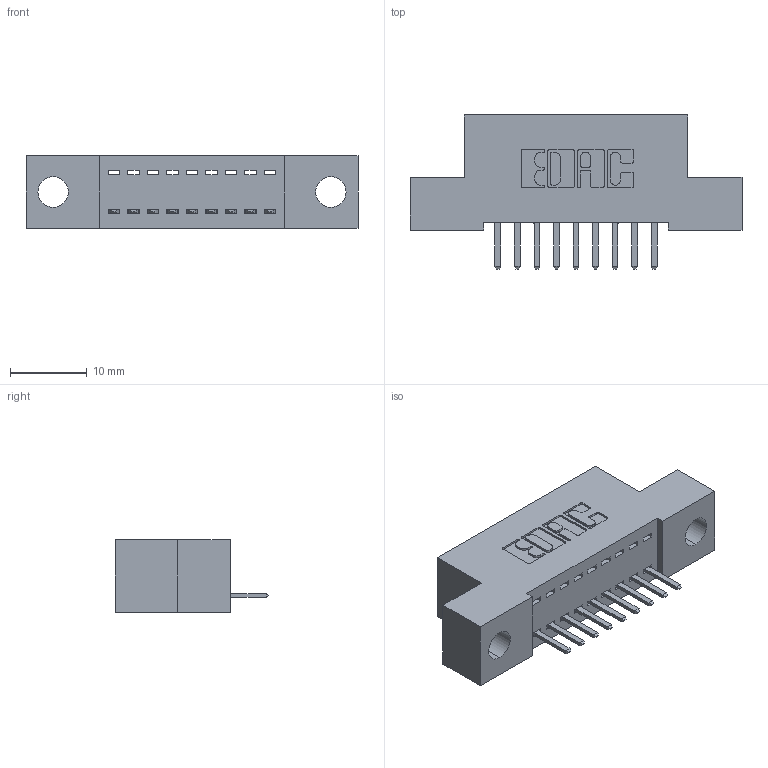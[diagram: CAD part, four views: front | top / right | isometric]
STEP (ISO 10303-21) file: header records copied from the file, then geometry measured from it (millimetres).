
FILE_DESCRIPTION (( 'STEP AP203' ), '1' );
FILE_NAME ('392-009-520-104.STEP', '2019-10-05T00:06:15', ( '' ), ( '' ), 'SwSTEP 2.0', 'SolidWorks 2016', '' );
FILE_SCHEMA (( 'CONFIG_CONTROL_DESIGN' ));
Length unit declared in the file: inch
Products named in the file (3): 342 Part_.156 TH; 345-292-001_345-293-120; 392-009-520-104
Assembly tree (10 placements, depth 2):
  392-009-520-104
    342 Part_.156 TH
    345-292-001_345-293-120  x9
Bounding box: 43.18 x 20.02 x 9.4 mm (x, y, z)
Volume: 3551.6 mm3; surface area: 4335.1 mm2
Topology: 10 solids, 10 shells, 668 faces, 1955 edges, 1278 vertices
Faces by surface type: plane 462, cylinder 206
Entity records: 9755 total; most frequent: CARTESIAN_POINT 1705, ORIENTED_EDGE 1638, DIRECTION 1493, EDGE_CURVE 819, VECTOR 687, LINE 687, VERTEX_POINT 542, AXIS2_PLACEMENT_3D 403
